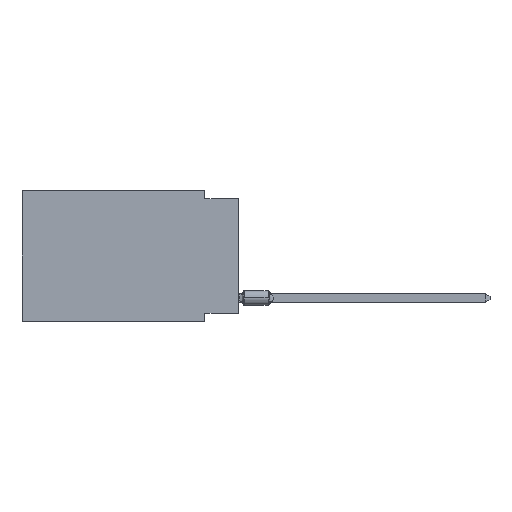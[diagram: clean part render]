
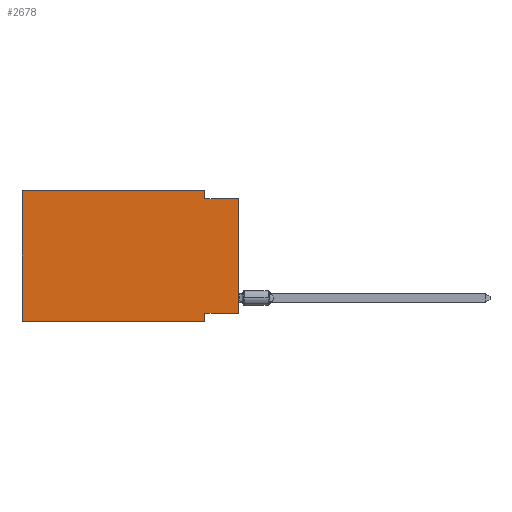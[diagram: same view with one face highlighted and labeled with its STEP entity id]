
A CAD part, left-side view. The second image highlights one B-rep face of the part: STEP entity #2678.
In plain terms, the highlighted planar face has unit normal (-1, 0, 0).
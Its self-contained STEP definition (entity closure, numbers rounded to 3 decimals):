
#1035 = VERTEX_POINT ( 'NONE', #14615 ) ;
#1527 = ORIENTED_EDGE ( 'NONE', *, *, #28231, .T. ) ;
#2181 = EDGE_CURVE ( 'NONE', #30312, #14636, #3506, .T. ) ;
#2678 = ADVANCED_FACE ( 'NONE', ( #29642 ), #29983, .F. ) ;
#3400 = VERTEX_POINT ( 'NONE', #32368 ) ;
#3506 = LINE ( 'NONE', #24598, #11540 ) ;
#3825 = CARTESIAN_POINT ( 'NONE',  ( 0., 0., -0.635 ) ) ;
#4355 = CARTESIAN_POINT ( 'NONE',  ( 0., 16.383, -9.906 ) ) ;
#5506 = VECTOR ( 'NONE', #27882, 1000. ) ;
#6430 = CARTESIAN_POINT ( 'NONE',  ( 0., 0., 0. ) ) ;
#6456 = CARTESIAN_POINT ( 'NONE',  ( 0., 16.383, 0. ) ) ;
#6779 = LINE ( 'NONE', #6430, #21965 ) ;
#7152 = DIRECTION ( 'NONE',  ( 0., 0., 1. ) ) ;
#8010 = CARTESIAN_POINT ( 'NONE',  ( 0., 0., -9.271 ) ) ;
#8197 = EDGE_CURVE ( 'NONE', #25729, #33828, #24602, .T. ) ;
#8420 = DIRECTION ( 'NONE',  ( 0., 0., -1. ) ) ;
#8813 = CARTESIAN_POINT ( 'NONE',  ( 0., 2.54, -9.271 ) ) ;
#9698 = VECTOR ( 'NONE', #7152, 1000. ) ;
#9767 = LINE ( 'NONE', #20495, #9698 ) ;
#11167 = LINE ( 'NONE', #21708, #26076 ) ;
#11540 = VECTOR ( 'NONE', #8420, 1000. ) ;
#11573 = AXIS2_PLACEMENT_3D ( 'NONE', #30336, #32977, #27010 ) ;
#13590 = EDGE_CURVE ( 'NONE', #3400, #24647, #19795, .T. ) ;
#13600 = VECTOR ( 'NONE', #18034, 1000. ) ;
#14398 = EDGE_LOOP ( 'NONE', ( #1527, #33142, #32254, #23799, #29229, #15105, #19064, #33400 ) ) ;
#14615 = CARTESIAN_POINT ( 'NONE',  ( 0., 16.383, -9.906 ) ) ;
#14636 = VERTEX_POINT ( 'NONE', #19734 ) ;
#15105 = ORIENTED_EDGE ( 'NONE', *, *, #23180, .T. ) ;
#15790 = VERTEX_POINT ( 'NONE', #8010 ) ;
#16330 = DIRECTION ( 'NONE',  ( 0., -1., 0. ) ) ;
#16497 = CARTESIAN_POINT ( 'NONE',  ( 0., 0., -0.635 ) ) ;
#16609 = DIRECTION ( 'NONE',  ( 0., 0., -1. ) ) ;
#17349 = DIRECTION ( 'NONE',  ( 0., 1., 0. ) ) ;
#17563 = VECTOR ( 'NONE', #16330, 1000. ) ;
#17685 = CARTESIAN_POINT ( 'NONE',  ( 0., 0., -9.271 ) ) ;
#17867 = LINE ( 'NONE', #17685, #28196 ) ;
#18034 = DIRECTION ( 'NONE',  ( 0., -1., 0. ) ) ;
#19064 = ORIENTED_EDGE ( 'NONE', *, *, #2181, .F. ) ;
#19194 = CARTESIAN_POINT ( 'NONE',  ( 0., 2.54, -0.635 ) ) ;
#19734 = CARTESIAN_POINT ( 'NONE',  ( 0., 2.54, -9.906 ) ) ;
#19795 = LINE ( 'NONE', #6456, #5506 ) ;
#20040 = EDGE_CURVE ( 'NONE', #24647, #25729, #11167, .T. ) ;
#20322 = LINE ( 'NONE', #4355, #13600 ) ;
#20495 = CARTESIAN_POINT ( 'NONE',  ( 0., 16.383, 0. ) ) ;
#21708 = CARTESIAN_POINT ( 'NONE',  ( 0., 2.54, 0. ) ) ;
#21965 = VECTOR ( 'NONE', #33795, 1000. ) ;
#23173 = EDGE_CURVE ( 'NONE', #15790, #30312, #17867, .T. ) ;
#23180 = EDGE_CURVE ( 'NONE', #1035, #14636, #20322, .T. ) ;
#23304 = EDGE_CURVE ( 'NONE', #1035, #3400, #9767, .T. ) ;
#23799 = ORIENTED_EDGE ( 'NONE', *, *, #13590, .F. ) ;
#24598 = CARTESIAN_POINT ( 'NONE',  ( 0., 2.54, -9.906 ) ) ;
#24602 = LINE ( 'NONE', #16497, #17563 ) ;
#24647 = VERTEX_POINT ( 'NONE', #32737 ) ;
#25729 = VERTEX_POINT ( 'NONE', #19194 ) ;
#26076 = VECTOR ( 'NONE', #16609, 1000. ) ;
#27010 = DIRECTION ( 'NONE',  ( 0., 0., -1. ) ) ;
#27882 = DIRECTION ( 'NONE',  ( 0., -1., 0. ) ) ;
#28196 = VECTOR ( 'NONE', #17349, 1000. ) ;
#28231 = EDGE_CURVE ( 'NONE', #15790, #33828, #6779, .T. ) ;
#29229 = ORIENTED_EDGE ( 'NONE', *, *, #23304, .F. ) ;
#29642 = FACE_OUTER_BOUND ( 'NONE', #14398, .T. ) ;
#29983 = PLANE ( 'NONE',  #11573 ) ;
#30312 = VERTEX_POINT ( 'NONE', #8813 ) ;
#30336 = CARTESIAN_POINT ( 'NONE',  ( 0., 16.383, 0. ) ) ;
#32254 = ORIENTED_EDGE ( 'NONE', *, *, #20040, .F. ) ;
#32368 = CARTESIAN_POINT ( 'NONE',  ( 0., 16.383, 0. ) ) ;
#32737 = CARTESIAN_POINT ( 'NONE',  ( 0., 2.54, 0. ) ) ;
#32977 = DIRECTION ( 'NONE',  ( 1., 0., 0. ) ) ;
#33142 = ORIENTED_EDGE ( 'NONE', *, *, #8197, .F. ) ;
#33400 = ORIENTED_EDGE ( 'NONE', *, *, #23173, .F. ) ;
#33795 = DIRECTION ( 'NONE',  ( 0., 0., 1. ) ) ;
#33828 = VERTEX_POINT ( 'NONE', #3825 ) ;
